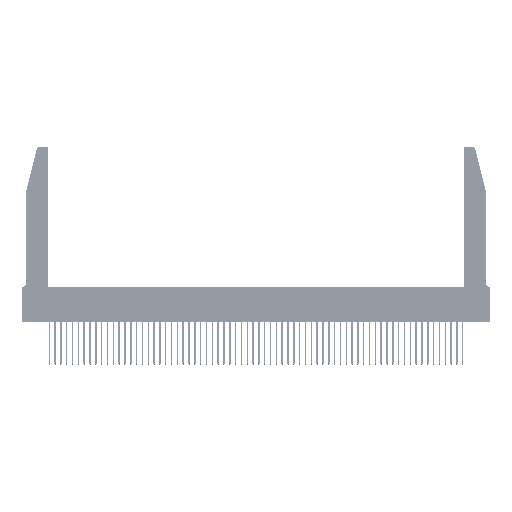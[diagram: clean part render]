
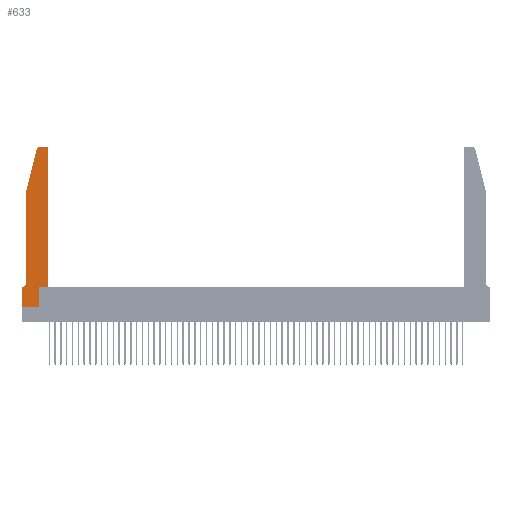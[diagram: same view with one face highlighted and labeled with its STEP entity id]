
A CAD part, top view. The second image highlights one B-rep face of the part: STEP entity #633.
In plain terms, the highlighted planar face has unit normal (0, 0, 1).
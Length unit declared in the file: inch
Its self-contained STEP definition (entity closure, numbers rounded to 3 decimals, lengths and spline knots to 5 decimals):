
#633 = ADVANCED_FACE ( 'NONE', ( #17546 ), #13268, .T. ) ;
#1193 = LINE ( 'NONE', #36631, #48889 ) ;
#1383 = LINE ( 'NONE', #22563, #33851 ) ;
#2153 = ORIENTED_EDGE ( 'NONE', *, *, #4762, .T. ) ;
#2298 = CIRCLE ( 'NONE', #50287, 0.03 ) ;
#2419 = CARTESIAN_POINT ( 'NONE',  ( 0.4205, 2.75, 0.37 ) ) ;
#3713 = VERTEX_POINT ( 'NONE', #22587 ) ;
#4362 = EDGE_CURVE ( 'NONE', #24946, #45593, #21477, .T. ) ;
#4736 = CARTESIAN_POINT ( 'NONE',  ( 0.2605, 2.75, 0.37 ) ) ;
#4762 = EDGE_CURVE ( 'NONE', #10940, #36228, #28306, .T. ) ;
#7296 = CARTESIAN_POINT ( 'NONE',  ( 0., 0.35, 0.37 ) ) ;
#7563 = VERTEX_POINT ( 'NONE', #25367 ) ;
#8160 = EDGE_LOOP ( 'NONE', ( #47798, #19875, #44728, #54502, #2153, #38640, #28614, #53886, #51781, #55552, #10164, #10107 ) ) ;
#9503 = CARTESIAN_POINT ( 'NONE',  ( 0.4505, 2.72, 0.37 ) ) ;
#9904 = CARTESIAN_POINT ( 'NONE',  ( 0.2865, 0., 0.37 ) ) ;
#10083 = VECTOR ( 'NONE', #49416, 39.37008 ) ;
#10107 = ORIENTED_EDGE ( 'NONE', *, *, #32255, .T. ) ;
#10164 = ORIENTED_EDGE ( 'NONE', *, *, #47405, .T. ) ;
#10940 = VERTEX_POINT ( 'NONE', #53660 ) ;
#11087 = DIRECTION ( 'NONE',  ( 1., 0., 0. ) ) ;
#12303 = DIRECTION ( 'NONE',  ( 1., 0., 0. ) ) ;
#12664 = CARTESIAN_POINT ( 'NONE',  ( 0., 0., 0.37 ) ) ;
#13099 = LINE ( 'NONE', #4736, #53900 ) ;
#13233 = DIRECTION ( 'NONE',  ( -1., 0., 0. ) ) ;
#13268 = PLANE ( 'NONE',  #50153 ) ;
#13288 = VERTEX_POINT ( 'NONE', #9904 ) ;
#13818 = CARTESIAN_POINT ( 'NONE',  ( 0.25487, 2.72718, 0.37 ) ) ;
#14463 = EDGE_CURVE ( 'NONE', #45593, #10940, #26840, .T. ) ;
#14612 = CARTESIAN_POINT ( 'NONE',  ( 0., 0., 0.37 ) ) ;
#15443 = CARTESIAN_POINT ( 'NONE',  ( 0.2865, 0.35, 0.37 ) ) ;
#15730 = LINE ( 'NONE', #15443, #45451 ) ;
#15932 = VECTOR ( 'NONE', #31251, 39.37008 ) ;
#17546 = FACE_OUTER_BOUND ( 'NONE', #8160, .T. ) ;
#17752 = DIRECTION ( 'NONE',  ( -1., 0., 0. ) ) ;
#17904 = CARTESIAN_POINT ( 'NONE',  ( 0.0755, 2., 0.37 ) ) ;
#19182 = AXIS2_PLACEMENT_3D ( 'NONE', #50165, #37568, #11087 ) ;
#19591 = CARTESIAN_POINT ( 'NONE',  ( 0.0755, 2., 0.37 ) ) ;
#19601 = DIRECTION ( 'NONE',  ( 1., 0., 0. ) ) ;
#19875 = ORIENTED_EDGE ( 'NONE', *, *, #45674, .T. ) ;
#19903 = AXIS2_PLACEMENT_3D ( 'NONE', #51719, #25188, #29654 ) ;
#20728 = VECTOR ( 'NONE', #56379, 39.37008 ) ;
#21284 = VECTOR ( 'NONE', #50223, 39.37008 ) ;
#21477 = LINE ( 'NONE', #17904, #15932 ) ;
#22563 = CARTESIAN_POINT ( 'NONE',  ( 0.0755, 0.35, 0.37 ) ) ;
#22587 = CARTESIAN_POINT ( 'NONE',  ( 0.4505, 0.35, 0.37 ) ) ;
#22767 = LINE ( 'NONE', #25867, #57122 ) ;
#23686 = EDGE_CURVE ( 'NONE', #13288, #38080, #15730, .T. ) ;
#24946 = VERTEX_POINT ( 'NONE', #13818 ) ;
#25188 = DIRECTION ( 'NONE',  ( 0., 0., -1. ) ) ;
#25367 = CARTESIAN_POINT ( 'NONE',  ( 0.284, 2.75, 0.37 ) ) ;
#25867 = CARTESIAN_POINT ( 'NONE',  ( 0.4505, 0.35, 0.37 ) ) ;
#26840 = LINE ( 'NONE', #55446, #21284 ) ;
#28306 = CIRCLE ( 'NONE', #19903, 0.07 ) ;
#28614 = ORIENTED_EDGE ( 'NONE', *, *, #54988, .T. ) ;
#29197 = EDGE_CURVE ( 'NONE', #52070, #7563, #13099, .T. ) ;
#29654 = DIRECTION ( 'NONE',  ( -1., 0., 0. ) ) ;
#30664 = DIRECTION ( 'NONE',  ( 0., 0., 1. ) ) ;
#31237 = DIRECTION ( 'NONE',  ( 1., 0., 0. ) ) ;
#31251 = DIRECTION ( 'NONE',  ( -0.239, -0.971, 0. ) ) ;
#32255 = EDGE_CURVE ( 'NONE', #52363, #52070, #2298, .T. ) ;
#32471 = LINE ( 'NONE', #12664, #20728 ) ;
#33054 = VERTEX_POINT ( 'NONE', #7296 ) ;
#33851 = VECTOR ( 'NONE', #17752, 39.37008 ) ;
#35674 = VERTEX_POINT ( 'NONE', #14612 ) ;
#36228 = VERTEX_POINT ( 'NONE', #48769 ) ;
#36631 = CARTESIAN_POINT ( 'NONE',  ( 0., 0., 0.37 ) ) ;
#37568 = DIRECTION ( 'NONE',  ( 0., 0., 1. ) ) ;
#38080 = VERTEX_POINT ( 'NONE', #46575 ) ;
#38640 = ORIENTED_EDGE ( 'NONE', *, *, #56491, .T. ) ;
#39162 = CARTESIAN_POINT ( 'NONE',  ( 0.4505, 0.35, 0.37 ) ) ;
#42687 = EDGE_CURVE ( 'NONE', #38080, #3713, #22767, .T. ) ;
#43413 = DIRECTION ( 'NONE',  ( 0., 0., 1. ) ) ;
#43647 = DIRECTION ( 'NONE',  ( 1., 0., 0. ) ) ;
#44728 = ORIENTED_EDGE ( 'NONE', *, *, #4362, .T. ) ;
#45451 = VECTOR ( 'NONE', #46558, 39.37008 ) ;
#45593 = VERTEX_POINT ( 'NONE', #19591 ) ;
#45674 = EDGE_CURVE ( 'NONE', #7563, #24946, #54592, .T. ) ;
#46558 = DIRECTION ( 'NONE',  ( 0., 1., 0. ) ) ;
#46575 = CARTESIAN_POINT ( 'NONE',  ( 0.2865, 0.35, 0.37 ) ) ;
#47405 = EDGE_CURVE ( 'NONE', #3713, #52363, #52328, .T. ) ;
#47571 = EDGE_CURVE ( 'NONE', #35674, #13288, #1193, .T. ) ;
#47798 = ORIENTED_EDGE ( 'NONE', *, *, #29197, .T. ) ;
#48769 = CARTESIAN_POINT ( 'NONE',  ( 0.0055, 0.35, 0.37 ) ) ;
#48889 = VECTOR ( 'NONE', #19601, 39.37008 ) ;
#49416 = DIRECTION ( 'NONE',  ( 0., 1., 0. ) ) ;
#50153 = AXIS2_PLACEMENT_3D ( 'NONE', #52734, #30664, #31237 ) ;
#50165 = CARTESIAN_POINT ( 'NONE',  ( 0.284, 2.72, 0.37 ) ) ;
#50223 = DIRECTION ( 'NONE',  ( 0., -1., 0. ) ) ;
#50287 = AXIS2_PLACEMENT_3D ( 'NONE', #56777, #43413, #12303 ) ;
#51719 = CARTESIAN_POINT ( 'NONE',  ( 0.0055, 0.42, 0.37 ) ) ;
#51781 = ORIENTED_EDGE ( 'NONE', *, *, #23686, .T. ) ;
#52070 = VERTEX_POINT ( 'NONE', #2419 ) ;
#52328 = LINE ( 'NONE', #39162, #10083 ) ;
#52363 = VERTEX_POINT ( 'NONE', #9503 ) ;
#52734 = CARTESIAN_POINT ( 'NONE',  ( 0., 0.35, 0.37 ) ) ;
#53660 = CARTESIAN_POINT ( 'NONE',  ( 0.0755, 0.42, 0.37 ) ) ;
#53886 = ORIENTED_EDGE ( 'NONE', *, *, #47571, .T. ) ;
#53900 = VECTOR ( 'NONE', #13233, 39.37008 ) ;
#54502 = ORIENTED_EDGE ( 'NONE', *, *, #14463, .T. ) ;
#54592 = CIRCLE ( 'NONE', #19182, 0.03 ) ;
#54988 = EDGE_CURVE ( 'NONE', #33054, #35674, #32471, .T. ) ;
#55446 = CARTESIAN_POINT ( 'NONE',  ( 0.0755, 2., 0.37 ) ) ;
#55552 = ORIENTED_EDGE ( 'NONE', *, *, #42687, .T. ) ;
#56379 = DIRECTION ( 'NONE',  ( 0., -1., 0. ) ) ;
#56491 = EDGE_CURVE ( 'NONE', #36228, #33054, #1383, .T. ) ;
#56777 = CARTESIAN_POINT ( 'NONE',  ( 0.4205, 2.72, 0.37 ) ) ;
#57122 = VECTOR ( 'NONE', #43647, 39.37008 ) ;
